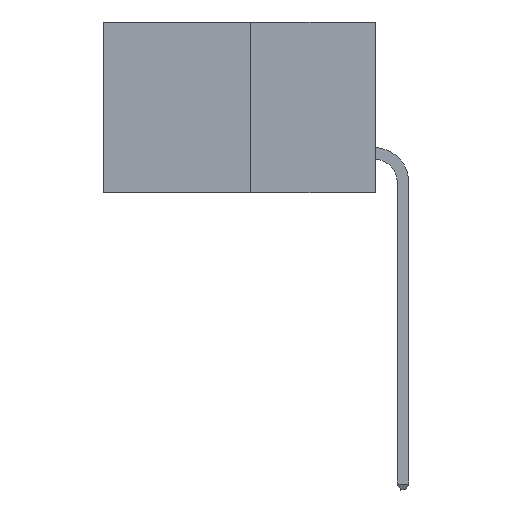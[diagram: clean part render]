
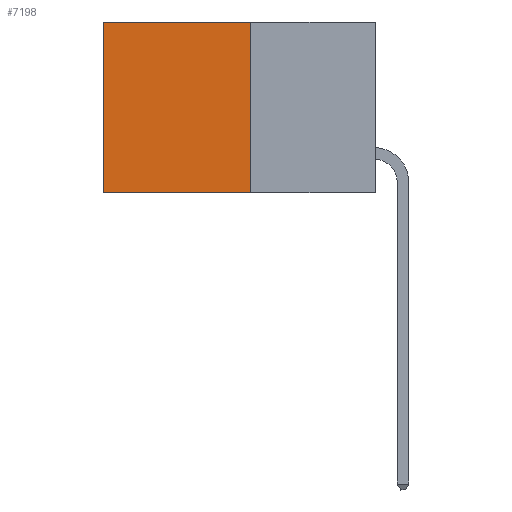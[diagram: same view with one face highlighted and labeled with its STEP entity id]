
A CAD part, left-side view. The second image highlights one B-rep face of the part: STEP entity #7198.
In plain terms, the highlighted planar face has unit normal (-1, 0, 0).
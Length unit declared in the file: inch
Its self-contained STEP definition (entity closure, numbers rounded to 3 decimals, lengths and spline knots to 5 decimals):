
#504 = ORIENTED_EDGE ( 'NONE', *, *, #5337, .F. ) ;
#603 = CARTESIAN_POINT ( 'NONE',  ( 0.277, 0.27, -0.37 ) ) ;
#816 = VERTEX_POINT ( 'NONE', #3433 ) ;
#1101 = VECTOR ( 'NONE', #7267, 39.37008 ) ;
#1274 = AXIS2_PLACEMENT_3D ( 'NONE', #2555, #10724, #5904 ) ;
#1581 = VERTEX_POINT ( 'NONE', #9588 ) ;
#2376 = EDGE_CURVE ( 'NONE', #1581, #6107, #8460, .T. ) ;
#2555 = CARTESIAN_POINT ( 'NONE',  ( 0.277, 0.27, -0.37 ) ) ;
#2665 = ORIENTED_EDGE ( 'NONE', *, *, #2376, .F. ) ;
#2799 = CARTESIAN_POINT ( 'NONE',  ( 0.277, 0.59, -0.37 ) ) ;
#3433 = CARTESIAN_POINT ( 'NONE',  ( 0.277, 0.59, 0. ) ) ;
#3832 = CARTESIAN_POINT ( 'NONE',  ( 0.277, 0.59, -0.37 ) ) ;
#4652 = DIRECTION ( 'NONE',  ( 0., 0., -1. ) ) ;
#4968 = CARTESIAN_POINT ( 'NONE',  ( 0.277, 0.27, -0.37 ) ) ;
#5228 = VECTOR ( 'NONE', #4652, 39.37008 ) ;
#5337 = EDGE_CURVE ( 'NONE', #6107, #7375, #9497, .T. ) ;
#5554 = EDGE_LOOP ( 'NONE', ( #9336, #504, #2665, #8147 ) ) ;
#5866 = LINE ( 'NONE', #8866, #1101 ) ;
#5904 = DIRECTION ( 'NONE',  ( 0., 0., -1. ) ) ;
#6107 = VERTEX_POINT ( 'NONE', #4968 ) ;
#6248 = CARTESIAN_POINT ( 'NONE',  ( 0.277, 0.27, -0.37 ) ) ;
#6264 = VECTOR ( 'NONE', #9138, 39.37008 ) ;
#6704 = PLANE ( 'NONE',  #1274 ) ;
#7198 = ADVANCED_FACE ( 'NONE', ( #7977 ), #6704, .F. ) ;
#7267 = DIRECTION ( 'NONE',  ( 0., 1., 0. ) ) ;
#7375 = VERTEX_POINT ( 'NONE', #2799 ) ;
#7379 = VECTOR ( 'NONE', #8960, 39.37008 ) ;
#7448 = LINE ( 'NONE', #3832, #5228 ) ;
#7977 = FACE_OUTER_BOUND ( 'NONE', #5554, .T. ) ;
#8147 = ORIENTED_EDGE ( 'NONE', *, *, #10192, .T. ) ;
#8149 = EDGE_CURVE ( 'NONE', #816, #7375, #7448, .T. ) ;
#8460 = LINE ( 'NONE', #6248, #6264 ) ;
#8866 = CARTESIAN_POINT ( 'NONE',  ( 0.277, 0.27, 0. ) ) ;
#8960 = DIRECTION ( 'NONE',  ( 0., 1., 0. ) ) ;
#9138 = DIRECTION ( 'NONE',  ( 0., 0., -1. ) ) ;
#9336 = ORIENTED_EDGE ( 'NONE', *, *, #8149, .T. ) ;
#9497 = LINE ( 'NONE', #603, #7379 ) ;
#9588 = CARTESIAN_POINT ( 'NONE',  ( 0.277, 0.27, 0. ) ) ;
#10192 = EDGE_CURVE ( 'NONE', #1581, #816, #5866, .T. ) ;
#10724 = DIRECTION ( 'NONE',  ( 1., 0., 0. ) ) ;
